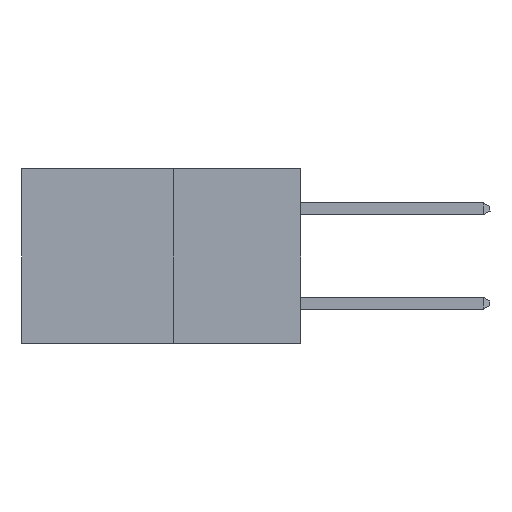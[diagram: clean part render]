
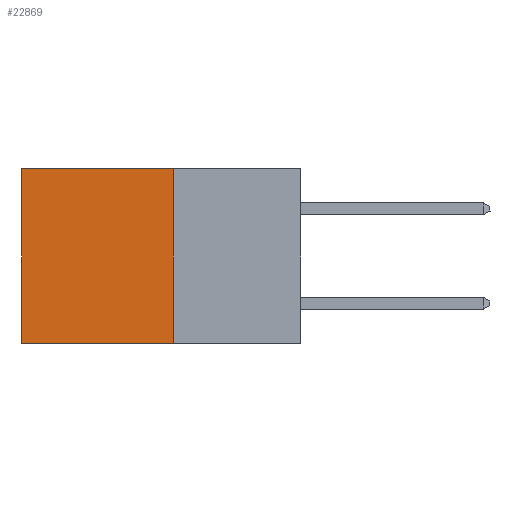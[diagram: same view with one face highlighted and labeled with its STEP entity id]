
A CAD part, left-side view. The second image highlights one B-rep face of the part: STEP entity #22869.
In plain terms, the highlighted planar face has unit normal (-1, 0, 0).
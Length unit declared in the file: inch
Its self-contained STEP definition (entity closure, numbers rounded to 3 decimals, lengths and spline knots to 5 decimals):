
#839 = VECTOR ( 'NONE', #3215, 39.37008 ) ;
#1313 = VECTOR ( 'NONE', #17389, 39.37008 ) ;
#1509 = CARTESIAN_POINT ( 'NONE',  ( 0.277, 0.59, -0.37 ) ) ;
#2583 = ORIENTED_EDGE ( 'NONE', *, *, #21550, .F. ) ;
#3215 = DIRECTION ( 'NONE',  ( 0., 1., 0. ) ) ;
#3436 = LINE ( 'NONE', #9012, #18327 ) ;
#5037 = CARTESIAN_POINT ( 'NONE',  ( 0.277, 0.27, -0.37 ) ) ;
#6653 = EDGE_CURVE ( 'NONE', #13436, #7501, #3436, .T. ) ;
#7501 = VERTEX_POINT ( 'NONE', #1509 ) ;
#7853 = VERTEX_POINT ( 'NONE', #14586 ) ;
#7954 = DIRECTION ( 'NONE',  ( 0., 0., -1. ) ) ;
#7963 = EDGE_CURVE ( 'NONE', #20620, #7501, #11261, .T. ) ;
#9012 = CARTESIAN_POINT ( 'NONE',  ( 0.277, 0.59, -0.37 ) ) ;
#9651 = ORIENTED_EDGE ( 'NONE', *, *, #20473, .T. ) ;
#9822 = ORIENTED_EDGE ( 'NONE', *, *, #7963, .F. ) ;
#11041 = ORIENTED_EDGE ( 'NONE', *, *, #6653, .T. ) ;
#11261 = LINE ( 'NONE', #18666, #839 ) ;
#11482 = VECTOR ( 'NONE', #16277, 39.37008 ) ;
#11718 = LINE ( 'NONE', #15464, #1313 ) ;
#11786 = CARTESIAN_POINT ( 'NONE',  ( 0.277, 0.27, -0.37 ) ) ;
#12401 = EDGE_LOOP ( 'NONE', ( #11041, #9822, #2583, #9651 ) ) ;
#13436 = VERTEX_POINT ( 'NONE', #23226 ) ;
#14586 = CARTESIAN_POINT ( 'NONE',  ( 0.277, 0.27, 0. ) ) ;
#15464 = CARTESIAN_POINT ( 'NONE',  ( 0.277, 0.27, -0.37 ) ) ;
#15666 = PLANE ( 'NONE',  #18931 ) ;
#16001 = LINE ( 'NONE', #23945, #11482 ) ;
#16277 = DIRECTION ( 'NONE',  ( 0., 1., 0. ) ) ;
#17389 = DIRECTION ( 'NONE',  ( 0., 0., -1. ) ) ;
#18327 = VECTOR ( 'NONE', #22449, 39.37008 ) ;
#18527 = FACE_OUTER_BOUND ( 'NONE', #12401, .T. ) ;
#18666 = CARTESIAN_POINT ( 'NONE',  ( 0.277, 0.27, -0.37 ) ) ;
#18931 = AXIS2_PLACEMENT_3D ( 'NONE', #11786, #19489, #7954 ) ;
#19489 = DIRECTION ( 'NONE',  ( 1., 0., 0. ) ) ;
#20473 = EDGE_CURVE ( 'NONE', #7853, #13436, #16001, .T. ) ;
#20620 = VERTEX_POINT ( 'NONE', #5037 ) ;
#21550 = EDGE_CURVE ( 'NONE', #7853, #20620, #11718, .T. ) ;
#22449 = DIRECTION ( 'NONE',  ( 0., 0., -1. ) ) ;
#22869 = ADVANCED_FACE ( 'NONE', ( #18527 ), #15666, .F. ) ;
#23226 = CARTESIAN_POINT ( 'NONE',  ( 0.277, 0.59, 0. ) ) ;
#23945 = CARTESIAN_POINT ( 'NONE',  ( 0.277, 0.27, 0. ) ) ;
